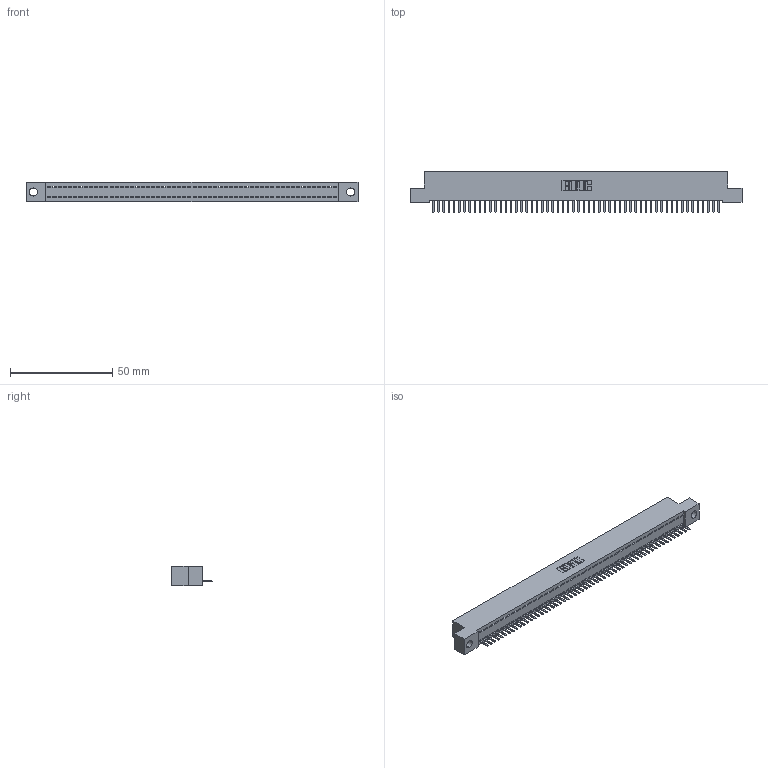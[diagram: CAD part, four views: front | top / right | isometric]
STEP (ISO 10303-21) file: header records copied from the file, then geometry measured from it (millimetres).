
FILE_DESCRIPTION (( 'STEP AP203' ), '1' );
FILE_NAME ('342-056-520-104.STEP', '2018-08-13T02:10:04', ( '' ), ( '' ), 'SwSTEP 2.0', 'SolidWorks 2016', '' );
FILE_SCHEMA (( 'CONFIG_CONTROL_DESIGN' ));
Length unit declared in the file: inch
Products named in the file (3): 342-056-520-104; 342 Part_.156 TH; 345-292-001_345-293-120
Assembly tree (57 placements, depth 2):
  342-056-520-104
    342 Part_.156 TH
    345-292-001_345-293-120  x56
Bounding box: 162.56 x 20.02 x 9.4 mm (x, y, z)
Volume: 14056.7 mm3; surface area: 20206.6 mm2
Topology: 57 solids, 57 shells, 3582 faces, 10603 edges, 6918 vertices
Faces by surface type: plane 2530, cylinder 1052
Entity records: 32409 total; most frequent: CARTESIAN_POINT 5606, ORIENTED_EDGE 5586, DIRECTION 4689, EDGE_CURVE 2793, LINE 2661, VECTOR 2661, VERTEX_POINT 1858, AXIS2_PLACEMENT_3D 1014
